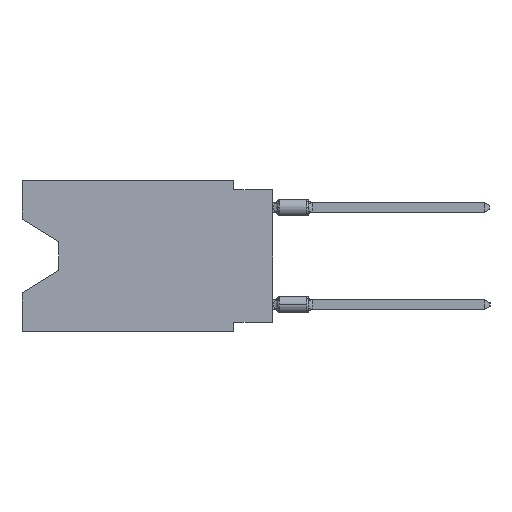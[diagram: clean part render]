
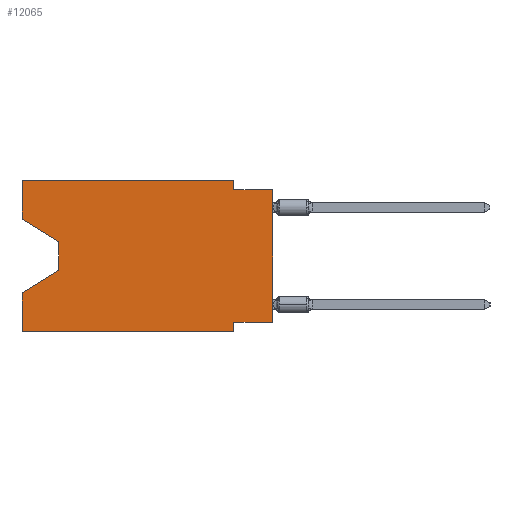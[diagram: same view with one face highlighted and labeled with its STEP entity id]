
A CAD part, left-side view. The second image highlights one B-rep face of the part: STEP entity #12065.
In plain terms, the highlighted planar face has unit normal (-1, 0, 0).
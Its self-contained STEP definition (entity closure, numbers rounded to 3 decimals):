
#1104 = VECTOR ( 'NONE', #5191, 1000. ) ;
#1952 = VERTEX_POINT ( 'NONE', #17123 ) ;
#2325 = VERTEX_POINT ( 'NONE', #32717 ) ;
#2863 = CARTESIAN_POINT ( 'NONE',  ( 0., 2.54, -0.635 ) ) ;
#2946 = VERTEX_POINT ( 'NONE', #13173 ) ;
#3162 = VERTEX_POINT ( 'NONE', #14116 ) ;
#3346 = AXIS2_PLACEMENT_3D ( 'NONE', #13270, #19294, #10852 ) ;
#4293 = EDGE_CURVE ( 'NONE', #15916, #37816, #9925, .T. ) ;
#5191 = DIRECTION ( 'NONE',  ( 0., 0., -1. ) ) ;
#5356 = EDGE_CURVE ( 'NONE', #24507, #25990, #23627, .T. ) ;
#6178 = CARTESIAN_POINT ( 'NONE',  ( 0., 13.97, -4.013 ) ) ;
#6179 = CARTESIAN_POINT ( 'NONE',  ( 0., 0., 0. ) ) ;
#6799 = VECTOR ( 'NONE', #15383, 1000. ) ;
#6907 = ORIENTED_EDGE ( 'NONE', *, *, #18252, .F. ) ;
#6994 = EDGE_CURVE ( 'NONE', #3162, #15916, #22288, .T. ) ;
#7105 = DIRECTION ( 'NONE',  ( 0., 0., -1. ) ) ;
#7610 = CARTESIAN_POINT ( 'NONE',  ( 0., 16.383, 0. ) ) ;
#7735 = ORIENTED_EDGE ( 'NONE', *, *, #10952, .F. ) ;
#7798 = DIRECTION ( 'NONE',  ( 0., 0., 1. ) ) ;
#9296 = CARTESIAN_POINT ( 'NONE',  ( 0., 0., -0.635 ) ) ;
#9444 = DIRECTION ( 'NONE',  ( 0., -1., 0. ) ) ;
#9839 = ORIENTED_EDGE ( 'NONE', *, *, #22733, .F. ) ;
#9925 = LINE ( 'NONE', #18734, #10615 ) ;
#10291 = VECTOR ( 'NONE', #7798, 1000. ) ;
#10540 = LINE ( 'NONE', #25776, #23249 ) ;
#10615 = VECTOR ( 'NONE', #7105, 1000. ) ;
#10852 = DIRECTION ( 'NONE',  ( 0., 0., -1. ) ) ;
#10952 = EDGE_CURVE ( 'NONE', #2946, #24507, #22229, .T. ) ;
#12065 = ADVANCED_FACE ( 'NONE', ( #16279 ), #37742, .F. ) ;
#12235 = VERTEX_POINT ( 'NONE', #17448 ) ;
#12631 = CARTESIAN_POINT ( 'NONE',  ( 0., 2.54, -9.906 ) ) ;
#12904 = ORIENTED_EDGE ( 'NONE', *, *, #39623, .F. ) ;
#13173 = CARTESIAN_POINT ( 'NONE',  ( 0., 16.383, 0. ) ) ;
#13270 = CARTESIAN_POINT ( 'NONE',  ( 0., 16.383, 0. ) ) ;
#14116 = CARTESIAN_POINT ( 'NONE',  ( 0., 16.383, -2.546 ) ) ;
#14281 = VERTEX_POINT ( 'NONE', #23629 ) ;
#14524 = ORIENTED_EDGE ( 'NONE', *, *, #5356, .F. ) ;
#14848 = EDGE_CURVE ( 'NONE', #37816, #12235, #24179, .T. ) ;
#15297 = LINE ( 'NONE', #9296, #25749 ) ;
#15383 = DIRECTION ( 'NONE',  ( 0., 0., 1. ) ) ;
#15760 = EDGE_CURVE ( 'NONE', #3162, #2946, #35870, .T. ) ;
#15916 = VERTEX_POINT ( 'NONE', #6178 ) ;
#16185 = CARTESIAN_POINT ( 'NONE',  ( 0., 2.54, -9.271 ) ) ;
#16279 = FACE_OUTER_BOUND ( 'NONE', #26034, .T. ) ;
#16405 = CARTESIAN_POINT ( 'NONE',  ( 0., 16.383, 0. ) ) ;
#16689 = DIRECTION ( 'NONE',  ( 0., 0., -1. ) ) ;
#17123 = CARTESIAN_POINT ( 'NONE',  ( 0., 0., -9.271 ) ) ;
#17294 = EDGE_CURVE ( 'NONE', #25990, #14281, #15297, .T. ) ;
#17448 = CARTESIAN_POINT ( 'NONE',  ( 0., 16.383, -7.36 ) ) ;
#17656 = ORIENTED_EDGE ( 'NONE', *, *, #21938, .T. ) ;
#17908 = ORIENTED_EDGE ( 'NONE', *, *, #14848, .T. ) ;
#18252 = EDGE_CURVE ( 'NONE', #1952, #31458, #10540, .T. ) ;
#18500 = VECTOR ( 'NONE', #37334, 1000. ) ;
#18734 = CARTESIAN_POINT ( 'NONE',  ( 0., 13.97, -4.013 ) ) ;
#18883 = CARTESIAN_POINT ( 'NONE',  ( 0., 16.383, -2.546 ) ) ;
#18946 = ORIENTED_EDGE ( 'NONE', *, *, #6994, .T. ) ;
#19294 = DIRECTION ( 'NONE',  ( 1., 0., 0. ) ) ;
#20431 = CARTESIAN_POINT ( 'NONE',  ( 0., 2.54, 0. ) ) ;
#21156 = ORIENTED_EDGE ( 'NONE', *, *, #17294, .F. ) ;
#21531 = DIRECTION ( 'NONE',  ( 0., -1., 0. ) ) ;
#21938 = EDGE_CURVE ( 'NONE', #2325, #30888, #27885, .T. ) ;
#22229 = LINE ( 'NONE', #16405, #31443 ) ;
#22288 = LINE ( 'NONE', #18883, #18500 ) ;
#22462 = CARTESIAN_POINT ( 'NONE',  ( 0., 16.383, -9.906 ) ) ;
#22486 = VECTOR ( 'NONE', #36413, 1000. ) ;
#22720 = LINE ( 'NONE', #31945, #34831 ) ;
#22733 = EDGE_CURVE ( 'NONE', #31458, #30888, #22720, .T. ) ;
#23249 = VECTOR ( 'NONE', #31396, 1000. ) ;
#23518 = ORIENTED_EDGE ( 'NONE', *, *, #4293, .T. ) ;
#23627 = LINE ( 'NONE', #20431, #1104 ) ;
#23629 = CARTESIAN_POINT ( 'NONE',  ( 0., 0., -0.635 ) ) ;
#24179 = LINE ( 'NONE', #39010, #22486 ) ;
#24507 = VERTEX_POINT ( 'NONE', #30821 ) ;
#24617 = LINE ( 'NONE', #6179, #6799 ) ;
#25412 = DIRECTION ( 'NONE',  ( 0., 0., 1. ) ) ;
#25607 = LINE ( 'NONE', #26004, #36140 ) ;
#25749 = VECTOR ( 'NONE', #21531, 1000. ) ;
#25776 = CARTESIAN_POINT ( 'NONE',  ( 0., 0., -9.271 ) ) ;
#25837 = VECTOR ( 'NONE', #9444, 1000. ) ;
#25990 = VERTEX_POINT ( 'NONE', #2863 ) ;
#26004 = CARTESIAN_POINT ( 'NONE',  ( 0., 16.383, 0. ) ) ;
#26034 = EDGE_LOOP ( 'NONE', ( #18946, #23518, #17908, #12904, #17656, #9839, #6907, #29479, #21156, #14524, #7735, #37454 ) ) ;
#27885 = LINE ( 'NONE', #22462, #25837 ) ;
#29479 = ORIENTED_EDGE ( 'NONE', *, *, #34732, .T. ) ;
#30821 = CARTESIAN_POINT ( 'NONE',  ( 0., 2.54, 0. ) ) ;
#30888 = VERTEX_POINT ( 'NONE', #12631 ) ;
#31396 = DIRECTION ( 'NONE',  ( 0., 1., 0. ) ) ;
#31440 = DIRECTION ( 'NONE',  ( 0., -1., 0. ) ) ;
#31443 = VECTOR ( 'NONE', #31440, 1000. ) ;
#31458 = VERTEX_POINT ( 'NONE', #16185 ) ;
#31945 = CARTESIAN_POINT ( 'NONE',  ( 0., 2.54, -9.906 ) ) ;
#32462 = CARTESIAN_POINT ( 'NONE',  ( 0., 13.97, -5.893 ) ) ;
#32717 = CARTESIAN_POINT ( 'NONE',  ( 0., 16.383, -9.906 ) ) ;
#34732 = EDGE_CURVE ( 'NONE', #1952, #14281, #24617, .T. ) ;
#34831 = VECTOR ( 'NONE', #16689, 1000. ) ;
#35870 = LINE ( 'NONE', #7610, #10291 ) ;
#36140 = VECTOR ( 'NONE', #25412, 1000. ) ;
#36413 = DIRECTION ( 'NONE',  ( 0., 0.855, -0.519 ) ) ;
#37334 = DIRECTION ( 'NONE',  ( 0., -0.855, -0.519 ) ) ;
#37454 = ORIENTED_EDGE ( 'NONE', *, *, #15760, .F. ) ;
#37742 = PLANE ( 'NONE',  #3346 ) ;
#37816 = VERTEX_POINT ( 'NONE', #32462 ) ;
#39010 = CARTESIAN_POINT ( 'NONE',  ( 0., 13.97, -5.893 ) ) ;
#39623 = EDGE_CURVE ( 'NONE', #2325, #12235, #25607, .T. ) ;
